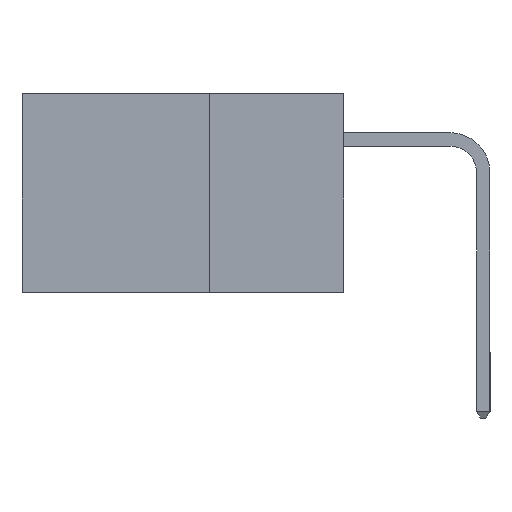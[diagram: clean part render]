
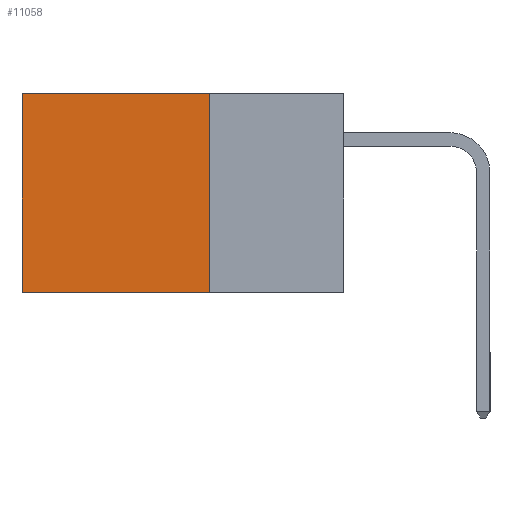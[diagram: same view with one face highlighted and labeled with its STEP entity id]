
A CAD part, left-side view. The second image highlights one B-rep face of the part: STEP entity #11058.
In plain terms, the highlighted planar face has unit normal (-1, 0, 0).
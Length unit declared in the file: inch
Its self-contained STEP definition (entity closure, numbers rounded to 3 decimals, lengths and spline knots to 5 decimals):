
#145 = VECTOR ( 'NONE', #5740, 39.37008 ) ;
#556 = LINE ( 'NONE', #4111, #3336 ) ;
#583 = VERTEX_POINT ( 'NONE', #7199 ) ;
#670 = ORIENTED_EDGE ( 'NONE', *, *, #1512, .F. ) ;
#916 = ORIENTED_EDGE ( 'NONE', *, *, #2126, .T. ) ;
#1139 = DIRECTION ( 'NONE',  ( 0., 1., 0. ) ) ;
#1181 = CARTESIAN_POINT ( 'NONE',  ( 0.298, 0.25, 0. ) ) ;
#1512 = EDGE_CURVE ( 'NONE', #6245, #8503, #2330, .T. ) ;
#1520 = CARTESIAN_POINT ( 'NONE',  ( 0.298, 0.6, -0.37 ) ) ;
#1705 = PLANE ( 'NONE',  #6080 ) ;
#1769 = DIRECTION ( 'NONE',  ( 0., 0., -1. ) ) ;
#1842 = CARTESIAN_POINT ( 'NONE',  ( 0.298, 0.25, -0.37 ) ) ;
#2110 = DIRECTION ( 'NONE',  ( 0., 0., -1. ) ) ;
#2126 = EDGE_CURVE ( 'NONE', #583, #8503, #556, .T. ) ;
#2240 = EDGE_CURVE ( 'NONE', #9042, #583, #11125, .T. ) ;
#2330 = LINE ( 'NONE', #1842, #145 ) ;
#2638 = DIRECTION ( 'NONE',  ( 1., 0., 0. ) ) ;
#3336 = VECTOR ( 'NONE', #1769, 39.37008 ) ;
#3747 = VECTOR ( 'NONE', #2110, 39.37008 ) ;
#4111 = CARTESIAN_POINT ( 'NONE',  ( 0.298, 0.6, 0. ) ) ;
#4486 = EDGE_CURVE ( 'NONE', #9042, #6245, #6478, .T. ) ;
#5740 = DIRECTION ( 'NONE',  ( 0., 1., 0. ) ) ;
#6080 = AXIS2_PLACEMENT_3D ( 'NONE', #8080, #2638, #8969 ) ;
#6245 = VERTEX_POINT ( 'NONE', #9459 ) ;
#6269 = ORIENTED_EDGE ( 'NONE', *, *, #4486, .F. ) ;
#6478 = LINE ( 'NONE', #1181, #3747 ) ;
#6630 = EDGE_LOOP ( 'NONE', ( #916, #670, #6269, #7815 ) ) ;
#7199 = CARTESIAN_POINT ( 'NONE',  ( 0.298, 0.6, 0. ) ) ;
#7815 = ORIENTED_EDGE ( 'NONE', *, *, #2240, .T. ) ;
#7962 = FACE_OUTER_BOUND ( 'NONE', #6630, .T. ) ;
#8080 = CARTESIAN_POINT ( 'NONE',  ( 0.298, 0.25, 0. ) ) ;
#8503 = VERTEX_POINT ( 'NONE', #1520 ) ;
#8969 = DIRECTION ( 'NONE',  ( 0., 0., -1. ) ) ;
#9042 = VERTEX_POINT ( 'NONE', #10403 ) ;
#9459 = CARTESIAN_POINT ( 'NONE',  ( 0.298, 0.25, -0.37 ) ) ;
#9721 = CARTESIAN_POINT ( 'NONE',  ( 0.298, 0.25, 0. ) ) ;
#10403 = CARTESIAN_POINT ( 'NONE',  ( 0.298, 0.25, 0. ) ) ;
#10857 = VECTOR ( 'NONE', #1139, 39.37008 ) ;
#11058 = ADVANCED_FACE ( 'NONE', ( #7962 ), #1705, .F. ) ;
#11125 = LINE ( 'NONE', #9721, #10857 ) ;
